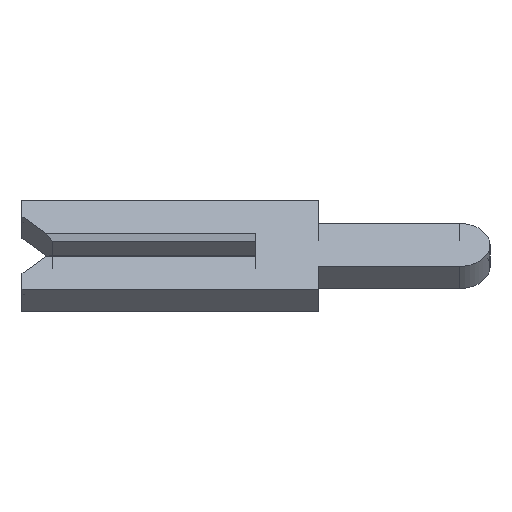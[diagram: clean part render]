
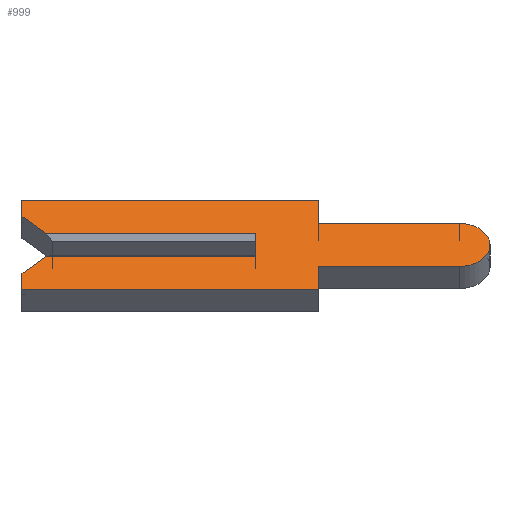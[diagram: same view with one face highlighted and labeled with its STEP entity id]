
A CAD part, left-side view. The second image highlights one B-rep face of the part: STEP entity #999.
In plain terms, the highlighted face is planar.
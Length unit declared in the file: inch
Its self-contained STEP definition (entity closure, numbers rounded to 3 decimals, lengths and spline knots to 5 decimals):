
#2 = EDGE_CURVE ( 'NONE', #1258, #949, #336, .T. ) ;
#8 = ORIENTED_EDGE ( 'NONE', *, *, #634, .F. ) ;
#11 = LINE ( 'NONE', #20, #455 ) ;
#18 = CARTESIAN_POINT ( 'NONE',  ( -0.01, -0.04, 0.0195 ) ) ;
#20 = CARTESIAN_POINT ( 'NONE',  ( -0.01, 0.1305, 0.0065 ) ) ;
#25 = ORIENTED_EDGE ( 'NONE', *, *, #2, .F. ) ;
#30 = CARTESIAN_POINT ( 'NONE',  ( -0.01, 0.1305, -0.0065 ) ) ;
#35 = DIRECTION ( 'NONE',  ( 0., 0., -1. ) ) ;
#37 = EDGE_CURVE ( 'NONE', #1567, #264, #1366, .T. ) ;
#57 = PLANE ( 'NONE',  #1168 ) ;
#88 = VERTEX_POINT ( 'NONE', #1299 ) ;
#105 = EDGE_CURVE ( 'NONE', #949, #264, #925, .T. ) ;
#132 = ORIENTED_EDGE ( 'NONE', *, *, #37, .T. ) ;
#155 = ORIENTED_EDGE ( 'NONE', *, *, #1285, .F. ) ;
#163 = DIRECTION ( 'NONE',  ( 0., -1., 0. ) ) ;
#167 = DIRECTION ( 'NONE',  ( 0., 0., -1. ) ) ;
#185 = VECTOR ( 'NONE', #1042, 39.37008 ) ;
#208 = VECTOR ( 'NONE', #516, 39.37008 ) ;
#210 = CARTESIAN_POINT ( 'NONE',  ( -0.01, 0.134, -0.01 ) ) ;
#218 = LINE ( 'NONE', #758, #275 ) ;
#230 = CARTESIAN_POINT ( 'NONE',  ( -0.01, -0.04, -0.0195 ) ) ;
#235 = VERTEX_POINT ( 'NONE', #1062 ) ;
#243 = LINE ( 'NONE', #714, #285 ) ;
#252 = CARTESIAN_POINT ( 'NONE',  ( -0.01, -0.04, -0.04 ) ) ;
#264 = VERTEX_POINT ( 'NONE', #1458 ) ;
#274 = VERTEX_POINT ( 'NONE', #802 ) ;
#275 = VECTOR ( 'NONE', #1272, 39.37008 ) ;
#281 = CIRCLE ( 'NONE', #1346, 0.0195 ) ;
#285 = VECTOR ( 'NONE', #35, 39.37008 ) ;
#290 = DIRECTION ( 'NONE',  ( 0., -0.707, 0.707 ) ) ;
#298 = VERTEX_POINT ( 'NONE', #1204 ) ;
#299 = DIRECTION ( 'NONE',  ( 0., 1., 0. ) ) ;
#300 = VECTOR ( 'NONE', #1278, 39.37008 ) ;
#301 = ORIENTED_EDGE ( 'NONE', *, *, #942, .F. ) ;
#311 = EDGE_CURVE ( 'NONE', #298, #1544, #497, .T. ) ;
#336 = LINE ( 'NONE', #1028, #185 ) ;
#368 = VECTOR ( 'NONE', #290, 39.37008 ) ;
#375 = CARTESIAN_POINT ( 'NONE',  ( -0.01, 0.15, 0.01 ) ) ;
#380 = DIRECTION ( 'NONE',  ( 0., -1., 0. ) ) ;
#414 = LINE ( 'NONE', #953, #736 ) ;
#432 = ORIENTED_EDGE ( 'NONE', *, *, #1208, .F. ) ;
#440 = CARTESIAN_POINT ( 'NONE',  ( -0.01, 0.15, 0.04 ) ) ;
#455 = VECTOR ( 'NONE', #687, 39.37008 ) ;
#480 = CARTESIAN_POINT ( 'NONE',  ( -0.01, -0.04, 0.0195 ) ) ;
#484 = EDGE_CURVE ( 'NONE', #1678, #1392, #414, .T. ) ;
#497 = LINE ( 'NONE', #928, #818 ) ;
#516 = DIRECTION ( 'NONE',  ( 0., 0., 1. ) ) ;
#580 = CARTESIAN_POINT ( 'NONE',  ( -0.01, 0.15, -0.026 ) ) ;
#594 = CARTESIAN_POINT ( 'NONE',  ( -0.01, -0.1305, 0. ) ) ;
#597 = CARTESIAN_POINT ( 'NONE',  ( -0.01, 0., -0.01 ) ) ;
#634 = EDGE_CURVE ( 'NONE', #1567, #1105, #11, .T. ) ;
#647 = VECTOR ( 'NONE', #163, 39.37008 ) ;
#687 = DIRECTION ( 'NONE',  ( 0., 0.707, 0.707 ) ) ;
#689 = ORIENTED_EDGE ( 'NONE', *, *, #763, .F. ) ;
#691 = VECTOR ( 'NONE', #986, 39.37008 ) ;
#714 = CARTESIAN_POINT ( 'NONE',  ( -0.01, -0.04, 0.04 ) ) ;
#730 = EDGE_CURVE ( 'NONE', #274, #1258, #1513, .T. ) ;
#736 = VECTOR ( 'NONE', #299, 39.37008 ) ;
#740 = ORIENTED_EDGE ( 'NONE', *, *, #484, .F. ) ;
#758 = CARTESIAN_POINT ( 'NONE',  ( -0.01, -0.04, -0.04 ) ) ;
#763 = EDGE_CURVE ( 'NONE', #88, #298, #281, .T. ) ;
#769 = VERTEX_POINT ( 'NONE', #18 ) ;
#771 = LINE ( 'NONE', #480, #1035 ) ;
#775 = EDGE_CURVE ( 'NONE', #1689, #235, #780, .T. ) ;
#780 = LINE ( 'NONE', #440, #647 ) ;
#793 = LINE ( 'NONE', #977, #300 ) ;
#802 = CARTESIAN_POINT ( 'NONE',  ( -0.01, 0.15, -0.026 ) ) ;
#818 = VECTOR ( 'NONE', #1060, 39.37008 ) ;
#821 = CARTESIAN_POINT ( 'NONE',  ( -0.01, -0.1305, 0. ) ) ;
#822 = VECTOR ( 'NONE', #380, 39.37008 ) ;
#876 = ORIENTED_EDGE ( 'NONE', *, *, #1327, .F. ) ;
#925 = LINE ( 'NONE', #1050, #208 ) ;
#928 = CARTESIAN_POINT ( 'NONE',  ( -0.01, -0.04, -0.0195 ) ) ;
#934 = ORIENTED_EDGE ( 'NONE', *, *, #1130, .F. ) ;
#942 = EDGE_CURVE ( 'NONE', #1392, #274, #1300, .T. ) ;
#949 = VERTEX_POINT ( 'NONE', #597 ) ;
#953 = CARTESIAN_POINT ( 'NONE',  ( -0.01, 0.15, -0.04 ) ) ;
#977 = CARTESIAN_POINT ( 'NONE',  ( -0.01, 0.15, 0.026 ) ) ;
#986 = DIRECTION ( 'NONE',  ( 0., 0., 1. ) ) ;
#999 = ADVANCED_FACE ( 'NONE', ( #1123 ), #57, .F. ) ;
#1012 = ORIENTED_EDGE ( 'NONE', *, *, #311, .F. ) ;
#1020 = DIRECTION ( 'NONE',  ( 0., -1., 0. ) ) ;
#1028 = CARTESIAN_POINT ( 'NONE',  ( -0.01, -0.1305, -0.01 ) ) ;
#1035 = VECTOR ( 'NONE', #1020, 39.37008 ) ;
#1042 = DIRECTION ( 'NONE',  ( 0., -1., 0. ) ) ;
#1050 = CARTESIAN_POINT ( 'NONE',  ( -0.01, 0., 0.0065 ) ) ;
#1060 = DIRECTION ( 'NONE',  ( 0., 1., 0. ) ) ;
#1062 = CARTESIAN_POINT ( 'NONE',  ( -0.01, -0.04, 0.04 ) ) ;
#1105 = VERTEX_POINT ( 'NONE', #1378 ) ;
#1107 = DIRECTION ( 'NONE',  ( 1., 0., 0. ) ) ;
#1123 = FACE_OUTER_BOUND ( 'NONE', #1233, .T. ) ;
#1130 = EDGE_CURVE ( 'NONE', #235, #769, #243, .T. ) ;
#1168 = AXIS2_PLACEMENT_3D ( 'NONE', #594, #1107, #1241 ) ;
#1204 = CARTESIAN_POINT ( 'NONE',  ( -0.01, -0.1305, -0.0195 ) ) ;
#1208 = EDGE_CURVE ( 'NONE', #1105, #1689, #793, .T. ) ;
#1224 = DIRECTION ( 'NONE',  ( 1., 0., 0. ) ) ;
#1233 = EDGE_LOOP ( 'NONE', ( #132, #1246, #25, #1404, #301, #740, #155, #1012, #689, #876, #934, #1532, #432, #8 ) ) ;
#1241 = DIRECTION ( 'NONE',  ( 0., 0., -1. ) ) ;
#1246 = ORIENTED_EDGE ( 'NONE', *, *, #105, .F. ) ;
#1258 = VERTEX_POINT ( 'NONE', #210 ) ;
#1272 = DIRECTION ( 'NONE',  ( 0., 0., -1. ) ) ;
#1278 = DIRECTION ( 'NONE',  ( 0., 0., 1. ) ) ;
#1285 = EDGE_CURVE ( 'NONE', #1544, #1678, #218, .T. ) ;
#1299 = CARTESIAN_POINT ( 'NONE',  ( -0.01, -0.1305, 0.0195 ) ) ;
#1300 = LINE ( 'NONE', #580, #691 ) ;
#1327 = EDGE_CURVE ( 'NONE', #769, #88, #771, .T. ) ;
#1346 = AXIS2_PLACEMENT_3D ( 'NONE', #821, #1224, #167 ) ;
#1366 = LINE ( 'NONE', #375, #822 ) ;
#1378 = CARTESIAN_POINT ( 'NONE',  ( -0.01, 0.15, 0.026 ) ) ;
#1392 = VERTEX_POINT ( 'NONE', #1409 ) ;
#1404 = ORIENTED_EDGE ( 'NONE', *, *, #730, .F. ) ;
#1409 = CARTESIAN_POINT ( 'NONE',  ( -0.01, 0.15, -0.04 ) ) ;
#1458 = CARTESIAN_POINT ( 'NONE',  ( -0.01, 0., 0.01 ) ) ;
#1513 = LINE ( 'NONE', #30, #368 ) ;
#1532 = ORIENTED_EDGE ( 'NONE', *, *, #775, .F. ) ;
#1544 = VERTEX_POINT ( 'NONE', #230 ) ;
#1558 = CARTESIAN_POINT ( 'NONE',  ( -0.01, 0.15, 0.04 ) ) ;
#1567 = VERTEX_POINT ( 'NONE', #1682 ) ;
#1678 = VERTEX_POINT ( 'NONE', #252 ) ;
#1682 = CARTESIAN_POINT ( 'NONE',  ( -0.01, 0.134, 0.01 ) ) ;
#1689 = VERTEX_POINT ( 'NONE', #1558 ) ;
